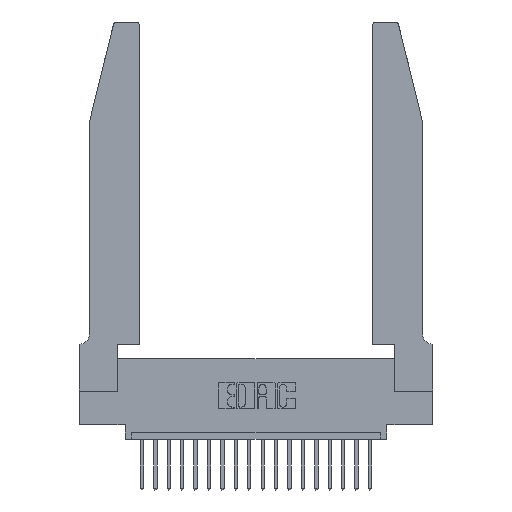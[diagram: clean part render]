
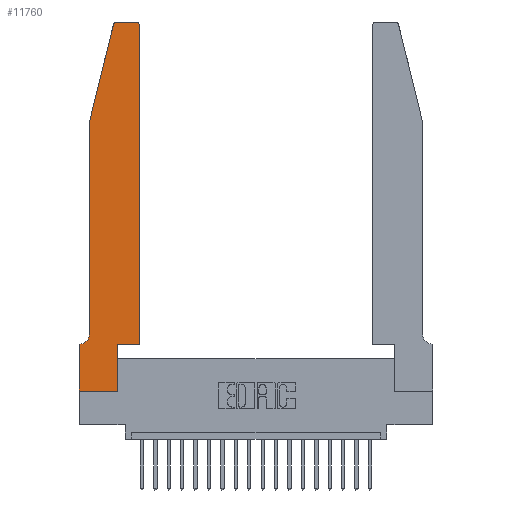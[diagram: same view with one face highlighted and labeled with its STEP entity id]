
A CAD part, top view. The second image highlights one B-rep face of the part: STEP entity #11760.
In plain terms, the highlighted planar face has unit normal (0, 0, 1).
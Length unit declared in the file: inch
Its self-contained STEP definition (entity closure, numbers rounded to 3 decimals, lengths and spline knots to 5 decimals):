
#14 = LINE ( 'NONE', #14275, #4749 ) ;
#193 = EDGE_CURVE ( 'NONE', #10361, #6123, #3556, .T. ) ;
#658 = CARTESIAN_POINT ( 'NONE',  ( 0., 0.35, 0.37 ) ) ;
#839 = EDGE_CURVE ( 'NONE', #6123, #4901, #14564, .T. ) ;
#1124 = ORIENTED_EDGE ( 'NONE', *, *, #6735, .T. ) ;
#1392 = DIRECTION ( 'NONE',  ( 0., 0., 1. ) ) ;
#1396 = VECTOR ( 'NONE', #17778, 39.37008 ) ;
#1510 = EDGE_LOOP ( 'NONE', ( #9114, #4932, #12201, #7314, #1606, #2483, #7555, #1124, #15603, #9169, #19487, #20402 ) ) ;
#1581 = CARTESIAN_POINT ( 'NONE',  ( 0.4505, 0.35, 0.37 ) ) ;
#1606 = ORIENTED_EDGE ( 'NONE', *, *, #13103, .T. ) ;
#1613 = DIRECTION ( 'NONE',  ( 0., -1., 0. ) ) ;
#2394 = EDGE_CURVE ( 'NONE', #4449, #10361, #10510, .T. ) ;
#2483 = ORIENTED_EDGE ( 'NONE', *, *, #9335, .T. ) ;
#2924 = DIRECTION ( 'NONE',  ( -1., 0., 0. ) ) ;
#3102 = EDGE_CURVE ( 'NONE', #13995, #4636, #18566, .T. ) ;
#3122 = VECTOR ( 'NONE', #13263, 39.37008 ) ;
#3379 = VECTOR ( 'NONE', #17994, 39.37008 ) ;
#3556 = LINE ( 'NONE', #20602, #17963 ) ;
#3595 = CARTESIAN_POINT ( 'NONE',  ( 0.0055, 0.35, 0.37 ) ) ;
#3824 = CARTESIAN_POINT ( 'NONE',  ( 0.0755, 2., 0.37 ) ) ;
#4043 = EDGE_CURVE ( 'NONE', #4636, #4449, #4440, .T. ) ;
#4440 = LINE ( 'NONE', #21266, #3379 ) ;
#4449 = VERTEX_POINT ( 'NONE', #11821 ) ;
#4636 = VERTEX_POINT ( 'NONE', #17499 ) ;
#4652 = CARTESIAN_POINT ( 'NONE',  ( 0.0055, 0.42, 0.37 ) ) ;
#4702 = VECTOR ( 'NONE', #18621, 39.37008 ) ;
#4749 = VECTOR ( 'NONE', #1613, 39.37008 ) ;
#4901 = VERTEX_POINT ( 'NONE', #13123 ) ;
#4932 = ORIENTED_EDGE ( 'NONE', *, *, #839, .T. ) ;
#5176 = CARTESIAN_POINT ( 'NONE',  ( 0., 0., 0.37 ) ) ;
#5709 = CARTESIAN_POINT ( 'NONE',  ( 0., 0., 0.37 ) ) ;
#5757 = EDGE_CURVE ( 'NONE', #12522, #17974, #14, .T. ) ;
#6123 = VERTEX_POINT ( 'NONE', #19735 ) ;
#6537 = CARTESIAN_POINT ( 'NONE',  ( 0.2865, 0.35, 0.37 ) ) ;
#6735 = EDGE_CURVE ( 'NONE', #12580, #13041, #15743, .T. ) ;
#6946 = LINE ( 'NONE', #6537, #1396 ) ;
#7314 = ORIENTED_EDGE ( 'NONE', *, *, #5757, .T. ) ;
#7555 = ORIENTED_EDGE ( 'NONE', *, *, #16928, .T. ) ;
#8041 = DIRECTION ( 'NONE',  ( 0., 0., 1. ) ) ;
#8246 = VECTOR ( 'NONE', #21223, 39.37008 ) ;
#8463 = CARTESIAN_POINT ( 'NONE',  ( 0.2865, 0.35, 0.37 ) ) ;
#9114 = ORIENTED_EDGE ( 'NONE', *, *, #193, .T. ) ;
#9169 = ORIENTED_EDGE ( 'NONE', *, *, #3102, .T. ) ;
#9335 = EDGE_CURVE ( 'NONE', #9939, #20812, #15874, .T. ) ;
#9697 = CARTESIAN_POINT ( 'NONE',  ( 0.4205, 2.75, 0.37 ) ) ;
#9936 = FACE_OUTER_BOUND ( 'NONE', #1510, .T. ) ;
#9939 = VERTEX_POINT ( 'NONE', #3595 ) ;
#10141 = DIRECTION ( 'NONE',  ( -1., 0., 0. ) ) ;
#10361 = VERTEX_POINT ( 'NONE', #9697 ) ;
#10510 = CIRCLE ( 'NONE', #17886, 0.03 ) ;
#11481 = DIRECTION ( 'NONE',  ( 1., 0., 0. ) ) ;
#11760 = ADVANCED_FACE ( 'NONE', ( #9936 ), #16860, .T. ) ;
#11821 = CARTESIAN_POINT ( 'NONE',  ( 0.4505, 2.72, 0.37 ) ) ;
#12201 = ORIENTED_EDGE ( 'NONE', *, *, #18039, .T. ) ;
#12522 = VERTEX_POINT ( 'NONE', #16067 ) ;
#12580 = VERTEX_POINT ( 'NONE', #5709 ) ;
#13041 = VERTEX_POINT ( 'NONE', #14926 ) ;
#13092 = DIRECTION ( 'NONE',  ( 0., 0., 1. ) ) ;
#13103 = EDGE_CURVE ( 'NONE', #17974, #9939, #21091, .T. ) ;
#13123 = CARTESIAN_POINT ( 'NONE',  ( 0.25487, 2.72718, 0.37 ) ) ;
#13151 = CARTESIAN_POINT ( 'NONE',  ( 0.0755, 0.35, 0.37 ) ) ;
#13263 = DIRECTION ( 'NONE',  ( 1., 0., 0. ) ) ;
#13302 = DIRECTION ( 'NONE',  ( 1., 0., 0. ) ) ;
#13995 = VERTEX_POINT ( 'NONE', #8463 ) ;
#14275 = CARTESIAN_POINT ( 'NONE',  ( 0.0755, 2., 0.37 ) ) ;
#14502 = AXIS2_PLACEMENT_3D ( 'NONE', #658, #13092, #20589 ) ;
#14564 = CIRCLE ( 'NONE', #14967, 0.03 ) ;
#14569 = VECTOR ( 'NONE', #20610, 39.37008 ) ;
#14785 = CARTESIAN_POINT ( 'NONE',  ( 0.284, 2.72, 0.37 ) ) ;
#14926 = CARTESIAN_POINT ( 'NONE',  ( 0.2865, 0., 0.37 ) ) ;
#14967 = AXIS2_PLACEMENT_3D ( 'NONE', #14785, #1392, #13302 ) ;
#15603 = ORIENTED_EDGE ( 'NONE', *, *, #18240, .T. ) ;
#15743 = LINE ( 'NONE', #20074, #4702 ) ;
#15874 = LINE ( 'NONE', #13151, #8246 ) ;
#16030 = LINE ( 'NONE', #5176, #21472 ) ;
#16067 = CARTESIAN_POINT ( 'NONE',  ( 0.0755, 2., 0.37 ) ) ;
#16383 = DIRECTION ( 'NONE',  ( 0., 0., -1. ) ) ;
#16812 = CARTESIAN_POINT ( 'NONE',  ( 0., 0.35, 0.37 ) ) ;
#16860 = PLANE ( 'NONE',  #14502 ) ;
#16928 = EDGE_CURVE ( 'NONE', #20812, #12580, #16030, .T. ) ;
#17499 = CARTESIAN_POINT ( 'NONE',  ( 0.4505, 0.35, 0.37 ) ) ;
#17778 = DIRECTION ( 'NONE',  ( 0., 1., 0. ) ) ;
#17886 = AXIS2_PLACEMENT_3D ( 'NONE', #21243, #8041, #11481 ) ;
#17963 = VECTOR ( 'NONE', #2924, 39.37008 ) ;
#17974 = VERTEX_POINT ( 'NONE', #19015 ) ;
#17994 = DIRECTION ( 'NONE',  ( 0., 1., 0. ) ) ;
#18039 = EDGE_CURVE ( 'NONE', #4901, #12522, #18698, .T. ) ;
#18240 = EDGE_CURVE ( 'NONE', #13041, #13995, #6946, .T. ) ;
#18566 = LINE ( 'NONE', #1581, #3122 ) ;
#18621 = DIRECTION ( 'NONE',  ( 1., 0., 0. ) ) ;
#18698 = LINE ( 'NONE', #3824, #14569 ) ;
#19015 = CARTESIAN_POINT ( 'NONE',  ( 0.0755, 0.42, 0.37 ) ) ;
#19487 = ORIENTED_EDGE ( 'NONE', *, *, #4043, .T. ) ;
#19735 = CARTESIAN_POINT ( 'NONE',  ( 0.284, 2.75, 0.37 ) ) ;
#20074 = CARTESIAN_POINT ( 'NONE',  ( 0., 0., 0.37 ) ) ;
#20190 = AXIS2_PLACEMENT_3D ( 'NONE', #4652, #16383, #10141 ) ;
#20402 = ORIENTED_EDGE ( 'NONE', *, *, #2394, .T. ) ;
#20485 = DIRECTION ( 'NONE',  ( 0., -1., 0. ) ) ;
#20589 = DIRECTION ( 'NONE',  ( 1., 0., 0. ) ) ;
#20602 = CARTESIAN_POINT ( 'NONE',  ( 0.2605, 2.75, 0.37 ) ) ;
#20610 = DIRECTION ( 'NONE',  ( -0.239, -0.971, 0. ) ) ;
#20812 = VERTEX_POINT ( 'NONE', #16812 ) ;
#21091 = CIRCLE ( 'NONE', #20190, 0.07 ) ;
#21223 = DIRECTION ( 'NONE',  ( -1., 0., 0. ) ) ;
#21243 = CARTESIAN_POINT ( 'NONE',  ( 0.4205, 2.72, 0.37 ) ) ;
#21266 = CARTESIAN_POINT ( 'NONE',  ( 0.4505, 0.35, 0.37 ) ) ;
#21472 = VECTOR ( 'NONE', #20485, 39.37008 ) ;
